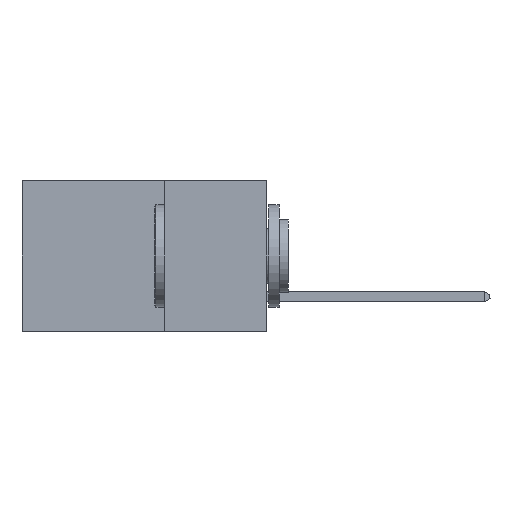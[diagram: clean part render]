
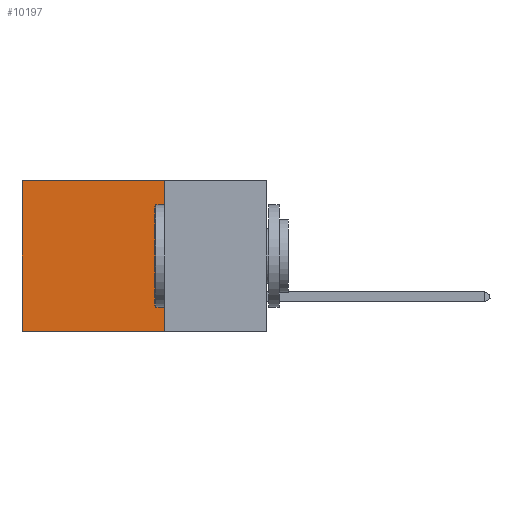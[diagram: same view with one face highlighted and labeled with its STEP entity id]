
A CAD part, left-side view. The second image highlights one B-rep face of the part: STEP entity #10197.
In plain terms, the highlighted planar face has unit normal (-1, 0, 0).
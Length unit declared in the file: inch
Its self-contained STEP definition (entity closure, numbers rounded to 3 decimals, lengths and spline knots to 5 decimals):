
#304 = CARTESIAN_POINT ( 'NONE',  ( 0.2875, 0.6, -0.37 ) ) ;
#554 = VERTEX_POINT ( 'NONE', #304 ) ;
#622 = EDGE_LOOP ( 'NONE', ( #20711, #16528, #15756, #13305 ) ) ;
#2103 = LINE ( 'NONE', #6726, #13143 ) ;
#2942 = CARTESIAN_POINT ( 'NONE',  ( 0.2875, 0.25, 0. ) ) ;
#4302 = EDGE_CURVE ( 'NONE', #15498, #13435, #6579, .T. ) ;
#4763 = LINE ( 'NONE', #20564, #12526 ) ;
#5026 = DIRECTION ( 'NONE',  ( 0., 0., -1. ) ) ;
#5196 = PLANE ( 'NONE',  #12453 ) ;
#5578 = DIRECTION ( 'NONE',  ( 0., 1., 0. ) ) ;
#5753 = FACE_OUTER_BOUND ( 'NONE', #622, .T. ) ;
#6579 = LINE ( 'NONE', #2942, #11386 ) ;
#6726 = CARTESIAN_POINT ( 'NONE',  ( 0.2875, 0.6, 0. ) ) ;
#7959 = DIRECTION ( 'NONE',  ( 0., 0., -1. ) ) ;
#8027 = CARTESIAN_POINT ( 'NONE',  ( 0.2875, 0.25, 0. ) ) ;
#8546 = DIRECTION ( 'NONE',  ( 1., 0., 0. ) ) ;
#8628 = EDGE_CURVE ( 'NONE', #15498, #14583, #19010, .T. ) ;
#10197 = ADVANCED_FACE ( 'NONE', ( #5753 ), #5196, .F. ) ;
#11386 = VECTOR ( 'NONE', #5578, 39.37008 ) ;
#12453 = AXIS2_PLACEMENT_3D ( 'NONE', #20598, #8546, #13742 ) ;
#12526 = VECTOR ( 'NONE', #20703, 39.37008 ) ;
#13143 = VECTOR ( 'NONE', #5026, 39.37008 ) ;
#13305 = ORIENTED_EDGE ( 'NONE', *, *, #4302, .T. ) ;
#13435 = VERTEX_POINT ( 'NONE', #14712 ) ;
#13742 = DIRECTION ( 'NONE',  ( 0., 0., -1. ) ) ;
#14583 = VERTEX_POINT ( 'NONE', #21742 ) ;
#14712 = CARTESIAN_POINT ( 'NONE',  ( 0.2875, 0.6, 0. ) ) ;
#15214 = VECTOR ( 'NONE', #7959, 39.37008 ) ;
#15498 = VERTEX_POINT ( 'NONE', #15719 ) ;
#15719 = CARTESIAN_POINT ( 'NONE',  ( 0.2875, 0.25, 0. ) ) ;
#15756 = ORIENTED_EDGE ( 'NONE', *, *, #8628, .F. ) ;
#16528 = ORIENTED_EDGE ( 'NONE', *, *, #20383, .F. ) ;
#17720 = EDGE_CURVE ( 'NONE', #13435, #554, #2103, .T. ) ;
#19010 = LINE ( 'NONE', #8027, #15214 ) ;
#20383 = EDGE_CURVE ( 'NONE', #14583, #554, #4763, .T. ) ;
#20564 = CARTESIAN_POINT ( 'NONE',  ( 0.2875, 0.25, -0.37 ) ) ;
#20598 = CARTESIAN_POINT ( 'NONE',  ( 0.2875, 0.25, 0. ) ) ;
#20703 = DIRECTION ( 'NONE',  ( 0., 1., 0. ) ) ;
#20711 = ORIENTED_EDGE ( 'NONE', *, *, #17720, .T. ) ;
#21742 = CARTESIAN_POINT ( 'NONE',  ( 0.2875, 0.25, -0.37 ) ) ;
